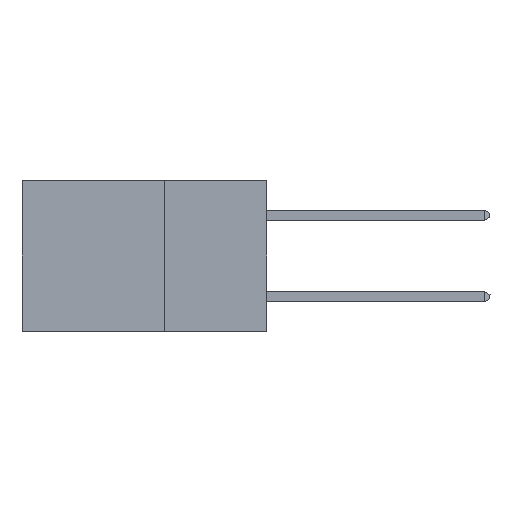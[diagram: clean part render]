
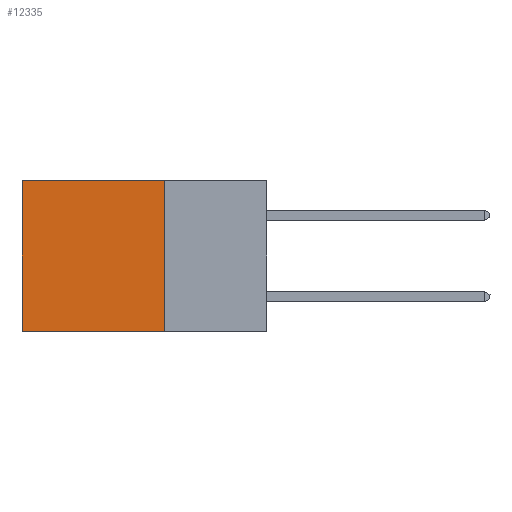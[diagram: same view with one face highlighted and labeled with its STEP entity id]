
A CAD part, left-side view. The second image highlights one B-rep face of the part: STEP entity #12335.
In plain terms, the highlighted planar face has unit normal (-1, 0, 0).
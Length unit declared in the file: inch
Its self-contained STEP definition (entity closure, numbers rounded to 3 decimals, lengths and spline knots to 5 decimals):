
#407 = LINE ( 'NONE', #7283, #10141 ) ;
#468 = DIRECTION ( 'NONE',  ( 1., 0., 0. ) ) ;
#516 = ORIENTED_EDGE ( 'NONE', *, *, #5486, .F. ) ;
#1451 = CARTESIAN_POINT ( 'NONE',  ( 0.2875, 0.25, -0.37 ) ) ;
#1524 = FACE_OUTER_BOUND ( 'NONE', #12801, .T. ) ;
#1728 = VECTOR ( 'NONE', #13036, 39.37008 ) ;
#2672 = EDGE_CURVE ( 'NONE', #11938, #5594, #10469, .T. ) ;
#3010 = DIRECTION ( 'NONE',  ( 0., 0., -1. ) ) ;
#3094 = AXIS2_PLACEMENT_3D ( 'NONE', #6947, #468, #4686 ) ;
#3642 = DIRECTION ( 'NONE',  ( 0., 1., 0. ) ) ;
#4266 = ORIENTED_EDGE ( 'NONE', *, *, #2672, .T. ) ;
#4686 = DIRECTION ( 'NONE',  ( 0., 0., -1. ) ) ;
#5332 = ORIENTED_EDGE ( 'NONE', *, *, #13545, .F. ) ;
#5486 = EDGE_CURVE ( 'NONE', #13717, #5594, #12291, .T. ) ;
#5594 = VERTEX_POINT ( 'NONE', #13612 ) ;
#5932 = CARTESIAN_POINT ( 'NONE',  ( 0.2875, 0.25, 0. ) ) ;
#5999 = VECTOR ( 'NONE', #3642, 39.37008 ) ;
#6947 = CARTESIAN_POINT ( 'NONE',  ( 0.2875, 0.25, 0. ) ) ;
#7283 = CARTESIAN_POINT ( 'NONE',  ( 0.2875, 0.25, 0. ) ) ;
#8668 = CARTESIAN_POINT ( 'NONE',  ( 0.2875, 0.25, 0. ) ) ;
#8997 = DIRECTION ( 'NONE',  ( 0., 0., -1. ) ) ;
#9098 = VECTOR ( 'NONE', #3010, 39.37008 ) ;
#9556 = ORIENTED_EDGE ( 'NONE', *, *, #11416, .T. ) ;
#10141 = VECTOR ( 'NONE', #8997, 39.37008 ) ;
#10199 = CARTESIAN_POINT ( 'NONE',  ( 0.2875, 0.6, 0. ) ) ;
#10469 = LINE ( 'NONE', #13775, #9098 ) ;
#11416 = EDGE_CURVE ( 'NONE', #11638, #11938, #12116, .T. ) ;
#11638 = VERTEX_POINT ( 'NONE', #5932 ) ;
#11847 = CARTESIAN_POINT ( 'NONE',  ( 0.2875, 0.25, -0.37 ) ) ;
#11938 = VERTEX_POINT ( 'NONE', #10199 ) ;
#12116 = LINE ( 'NONE', #8668, #1728 ) ;
#12291 = LINE ( 'NONE', #1451, #5999 ) ;
#12335 = ADVANCED_FACE ( 'NONE', ( #1524 ), #13206, .F. ) ;
#12801 = EDGE_LOOP ( 'NONE', ( #4266, #516, #5332, #9556 ) ) ;
#13036 = DIRECTION ( 'NONE',  ( 0., 1., 0. ) ) ;
#13206 = PLANE ( 'NONE',  #3094 ) ;
#13545 = EDGE_CURVE ( 'NONE', #11638, #13717, #407, .T. ) ;
#13612 = CARTESIAN_POINT ( 'NONE',  ( 0.2875, 0.6, -0.37 ) ) ;
#13717 = VERTEX_POINT ( 'NONE', #11847 ) ;
#13775 = CARTESIAN_POINT ( 'NONE',  ( 0.2875, 0.6, 0. ) ) ;
